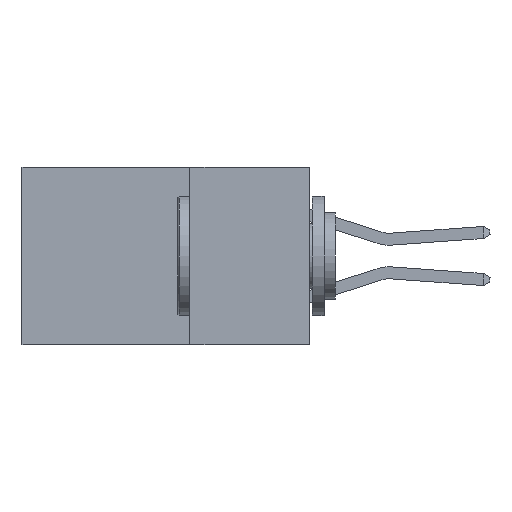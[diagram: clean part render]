
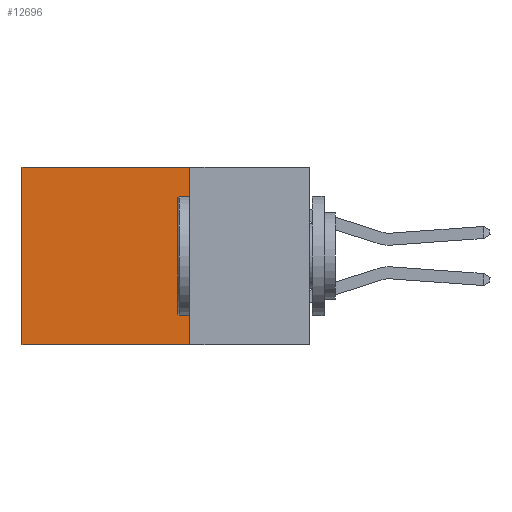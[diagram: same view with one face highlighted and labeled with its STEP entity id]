
A CAD part, left-side view. The second image highlights one B-rep face of the part: STEP entity #12696.
In plain terms, the highlighted planar face has unit normal (-1, 0, 0).
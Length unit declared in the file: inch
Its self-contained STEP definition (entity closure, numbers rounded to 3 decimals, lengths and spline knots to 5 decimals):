
#11 = VERTEX_POINT ( 'NONE', #3671 ) ;
#130 = DIRECTION ( 'NONE',  ( 0., 0., -1. ) ) ;
#265 = VERTEX_POINT ( 'NONE', #8502 ) ;
#319 = DIRECTION ( 'NONE',  ( 0., 1., 0. ) ) ;
#1609 = VECTOR ( 'NONE', #2117, 39.37008 ) ;
#1733 = FACE_OUTER_BOUND ( 'NONE', #5849, .T. ) ;
#2117 = DIRECTION ( 'NONE',  ( 0., 0., -1. ) ) ;
#3159 = EDGE_CURVE ( 'NONE', #9405, #10214, #12410, .T. ) ;
#3514 = DIRECTION ( 'NONE',  ( 0., 0., -1. ) ) ;
#3671 = CARTESIAN_POINT ( 'NONE',  ( 0.298, 0.6, 0. ) ) ;
#3916 = CARTESIAN_POINT ( 'NONE',  ( 0.298, 0.25, -0.37 ) ) ;
#4381 = LINE ( 'NONE', #8925, #7437 ) ;
#4535 = VECTOR ( 'NONE', #7645, 39.37008 ) ;
#4612 = LINE ( 'NONE', #6744, #8681 ) ;
#4909 = AXIS2_PLACEMENT_3D ( 'NONE', #9721, #6508, #130 ) ;
#5849 = EDGE_LOOP ( 'NONE', ( #12963, #7802, #7285, #9106 ) ) ;
#6508 = DIRECTION ( 'NONE',  ( 1., 0., 0. ) ) ;
#6744 = CARTESIAN_POINT ( 'NONE',  ( 0.298, 0.25, 0. ) ) ;
#7285 = ORIENTED_EDGE ( 'NONE', *, *, #3159, .F. ) ;
#7437 = VECTOR ( 'NONE', #3514, 39.37008 ) ;
#7483 = CARTESIAN_POINT ( 'NONE',  ( 0.298, 0.25, 0. ) ) ;
#7536 = EDGE_CURVE ( 'NONE', #11, #265, #4381, .T. ) ;
#7645 = DIRECTION ( 'NONE',  ( 0., 1., 0. ) ) ;
#7802 = ORIENTED_EDGE ( 'NONE', *, *, #8247, .F. ) ;
#8247 = EDGE_CURVE ( 'NONE', #10214, #265, #13482, .T. ) ;
#8502 = CARTESIAN_POINT ( 'NONE',  ( 0.298, 0.6, -0.37 ) ) ;
#8662 = PLANE ( 'NONE',  #4909 ) ;
#8681 = VECTOR ( 'NONE', #319, 39.37008 ) ;
#8889 = CARTESIAN_POINT ( 'NONE',  ( 0.298, 0.25, 0. ) ) ;
#8925 = CARTESIAN_POINT ( 'NONE',  ( 0.298, 0.6, 0. ) ) ;
#9106 = ORIENTED_EDGE ( 'NONE', *, *, #12246, .T. ) ;
#9405 = VERTEX_POINT ( 'NONE', #8889 ) ;
#9721 = CARTESIAN_POINT ( 'NONE',  ( 0.298, 0.25, 0. ) ) ;
#10214 = VERTEX_POINT ( 'NONE', #3916 ) ;
#12246 = EDGE_CURVE ( 'NONE', #9405, #11, #4612, .T. ) ;
#12410 = LINE ( 'NONE', #7483, #1609 ) ;
#12696 = ADVANCED_FACE ( 'NONE', ( #1733 ), #8662, .F. ) ;
#12963 = ORIENTED_EDGE ( 'NONE', *, *, #7536, .T. ) ;
#13023 = CARTESIAN_POINT ( 'NONE',  ( 0.298, 0.25, -0.37 ) ) ;
#13482 = LINE ( 'NONE', #13023, #4535 ) ;
